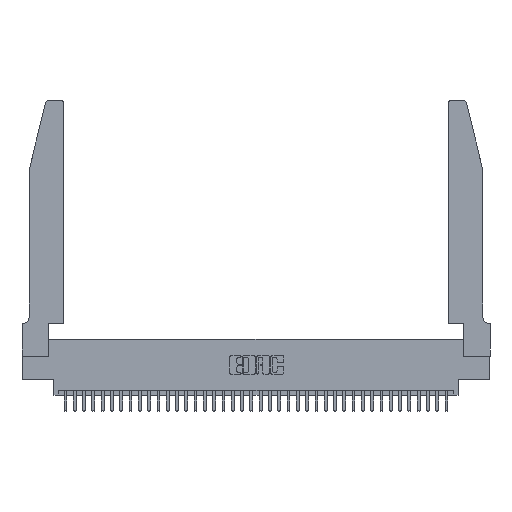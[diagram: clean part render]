
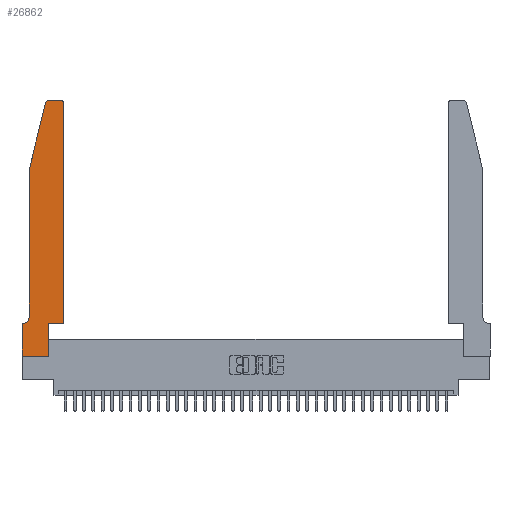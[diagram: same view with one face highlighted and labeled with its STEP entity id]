
A CAD part, top view. The second image highlights one B-rep face of the part: STEP entity #26862.
In plain terms, the highlighted planar face has unit normal (0, 0, 1).
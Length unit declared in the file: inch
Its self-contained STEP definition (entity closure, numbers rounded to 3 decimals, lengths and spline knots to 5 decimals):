
#395 = ORIENTED_EDGE ( 'NONE', *, *, #16836, .T. ) ;
#400 = VERTEX_POINT ( 'NONE', #13882 ) ;
#529 = CARTESIAN_POINT ( 'NONE',  ( 0.0755, 2., 0.37 ) ) ;
#575 = PLANE ( 'NONE',  #10011 ) ;
#700 = DIRECTION ( 'NONE',  ( 1., 0., 0. ) ) ;
#1542 = DIRECTION ( 'NONE',  ( 1., 0., 0. ) ) ;
#2435 = VECTOR ( 'NONE', #3295, 39.37008 ) ;
#2620 = VECTOR ( 'NONE', #33960, 39.37008 ) ;
#2962 = LINE ( 'NONE', #3647, #18760 ) ;
#3295 = DIRECTION ( 'NONE',  ( 0., -1., 0. ) ) ;
#3554 = CARTESIAN_POINT ( 'NONE',  ( 0.0055, 0.42, 0.37 ) ) ;
#3647 = CARTESIAN_POINT ( 'NONE',  ( 0., 0., 0.37 ) ) ;
#4243 = VECTOR ( 'NONE', #6695, 39.37008 ) ;
#4489 = VECTOR ( 'NONE', #28219, 39.37008 ) ;
#5082 = CARTESIAN_POINT ( 'NONE',  ( 0.0755, 0.42, 0.37 ) ) ;
#5367 = LINE ( 'NONE', #30087, #10593 ) ;
#5373 = CARTESIAN_POINT ( 'NONE',  ( 0.4505, 0.35, 0.37 ) ) ;
#5384 = VECTOR ( 'NONE', #25978, 39.37008 ) ;
#5911 = ORIENTED_EDGE ( 'NONE', *, *, #30360, .T. ) ;
#5937 = CARTESIAN_POINT ( 'NONE',  ( 0., 0.35, 0.37 ) ) ;
#6180 = ORIENTED_EDGE ( 'NONE', *, *, #32149, .T. ) ;
#6586 = DIRECTION ( 'NONE',  ( -1., 0., 0. ) ) ;
#6668 = DIRECTION ( 'NONE',  ( 0., -1., 0. ) ) ;
#6695 = DIRECTION ( 'NONE',  ( 0., 1., 0. ) ) ;
#6827 = CARTESIAN_POINT ( 'NONE',  ( 0.4505, 0.35, 0.37 ) ) ;
#6992 = CARTESIAN_POINT ( 'NONE',  ( 0.2865, 0., 0.37 ) ) ;
#8210 = CARTESIAN_POINT ( 'NONE',  ( 0.0755, 2., 0.37 ) ) ;
#8322 = CARTESIAN_POINT ( 'NONE',  ( 0.2865, 0.35, 0.37 ) ) ;
#8502 = VERTEX_POINT ( 'NONE', #5082 ) ;
#8760 = LINE ( 'NONE', #13748, #2620 ) ;
#8770 = CARTESIAN_POINT ( 'NONE',  ( 0., 0., 0.37 ) ) ;
#9893 = AXIS2_PLACEMENT_3D ( 'NONE', #12960, #33146, #15864 ) ;
#9924 = VERTEX_POINT ( 'NONE', #32906 ) ;
#10011 = AXIS2_PLACEMENT_3D ( 'NONE', #29972, #18523, #700 ) ;
#10066 = ORIENTED_EDGE ( 'NONE', *, *, #23446, .T. ) ;
#10461 = VERTEX_POINT ( 'NONE', #5937 ) ;
#10507 = LINE ( 'NONE', #23837, #2435 ) ;
#10521 = VERTEX_POINT ( 'NONE', #29562 ) ;
#10593 = VECTOR ( 'NONE', #27276, 39.37008 ) ;
#10937 = CARTESIAN_POINT ( 'NONE',  ( 0.4505, 0.35, 0.37 ) ) ;
#11650 = ORIENTED_EDGE ( 'NONE', *, *, #18277, .T. ) ;
#11879 = ORIENTED_EDGE ( 'NONE', *, *, #30148, .T. ) ;
#12250 = LINE ( 'NONE', #32814, #4243 ) ;
#12498 = LINE ( 'NONE', #10937, #4489 ) ;
#12588 = VERTEX_POINT ( 'NONE', #6992 ) ;
#12918 = LINE ( 'NONE', #8210, #20580 ) ;
#12960 = CARTESIAN_POINT ( 'NONE',  ( 0.284, 2.72, 0.37 ) ) ;
#13748 = CARTESIAN_POINT ( 'NONE',  ( 0.2605, 2.75, 0.37 ) ) ;
#13882 = CARTESIAN_POINT ( 'NONE',  ( 0., 0., 0.37 ) ) ;
#14014 = CARTESIAN_POINT ( 'NONE',  ( 0.4505, 2.72, 0.37 ) ) ;
#14274 = LINE ( 'NONE', #5373, #5384 ) ;
#14416 = FACE_OUTER_BOUND ( 'NONE', #36557, .T. ) ;
#15118 = VERTEX_POINT ( 'NONE', #31082 ) ;
#15179 = VERTEX_POINT ( 'NONE', #14014 ) ;
#15702 = EDGE_CURVE ( 'NONE', #23972, #27728, #12498, .T. ) ;
#15864 = DIRECTION ( 'NONE',  ( 1., 0., 0. ) ) ;
#16251 = ORIENTED_EDGE ( 'NONE', *, *, #22519, .T. ) ;
#16836 = EDGE_CURVE ( 'NONE', #27728, #15179, #14274, .T. ) ;
#17478 = EDGE_CURVE ( 'NONE', #400, #12588, #36845, .T. ) ;
#18226 = AXIS2_PLACEMENT_3D ( 'NONE', #3554, #24074, #6586 ) ;
#18277 = EDGE_CURVE ( 'NONE', #29444, #8502, #10507, .T. ) ;
#18523 = DIRECTION ( 'NONE',  ( 0., 0., 1. ) ) ;
#18760 = VECTOR ( 'NONE', #6668, 39.37008 ) ;
#19197 = CIRCLE ( 'NONE', #34561, 0.03 ) ;
#19300 = DIRECTION ( 'NONE',  ( 0., 0., 1. ) ) ;
#19609 = ORIENTED_EDGE ( 'NONE', *, *, #23746, .T. ) ;
#20580 = VECTOR ( 'NONE', #25808, 39.37008 ) ;
#22519 = EDGE_CURVE ( 'NONE', #8502, #27505, #29205, .T. ) ;
#23446 = EDGE_CURVE ( 'NONE', #10521, #29444, #12918, .T. ) ;
#23746 = EDGE_CURVE ( 'NONE', #27505, #10461, #5367, .T. ) ;
#23837 = CARTESIAN_POINT ( 'NONE',  ( 0.0755, 2., 0.37 ) ) ;
#23972 = VERTEX_POINT ( 'NONE', #8322 ) ;
#24074 = DIRECTION ( 'NONE',  ( 0., 0., -1. ) ) ;
#24427 = ORIENTED_EDGE ( 'NONE', *, *, #27918, .T. ) ;
#25443 = ORIENTED_EDGE ( 'NONE', *, *, #17478, .T. ) ;
#25808 = DIRECTION ( 'NONE',  ( -0.239, -0.971, 0. ) ) ;
#25978 = DIRECTION ( 'NONE',  ( 0., 1., 0. ) ) ;
#26862 = ADVANCED_FACE ( 'NONE', ( #14416 ), #575, .T. ) ;
#27276 = DIRECTION ( 'NONE',  ( -1., 0., 0. ) ) ;
#27505 = VERTEX_POINT ( 'NONE', #32841 ) ;
#27728 = VERTEX_POINT ( 'NONE', #6827 ) ;
#27918 = EDGE_CURVE ( 'NONE', #15118, #9924, #8760, .T. ) ;
#28201 = ORIENTED_EDGE ( 'NONE', *, *, #32871, .T. ) ;
#28219 = DIRECTION ( 'NONE',  ( 1., 0., 0. ) ) ;
#29205 = CIRCLE ( 'NONE', #18226, 0.07 ) ;
#29444 = VERTEX_POINT ( 'NONE', #529 ) ;
#29562 = CARTESIAN_POINT ( 'NONE',  ( 0.25487, 2.72718, 0.37 ) ) ;
#29972 = CARTESIAN_POINT ( 'NONE',  ( 0., 0.35, 0.37 ) ) ;
#30087 = CARTESIAN_POINT ( 'NONE',  ( 0.0755, 0.35, 0.37 ) ) ;
#30148 = EDGE_CURVE ( 'NONE', #10461, #400, #2962, .T. ) ;
#30360 = EDGE_CURVE ( 'NONE', #15179, #15118, #19197, .T. ) ;
#30411 = ORIENTED_EDGE ( 'NONE', *, *, #15702, .T. ) ;
#31082 = CARTESIAN_POINT ( 'NONE',  ( 0.4205, 2.75, 0.37 ) ) ;
#32149 = EDGE_CURVE ( 'NONE', #12588, #23972, #12250, .T. ) ;
#32814 = CARTESIAN_POINT ( 'NONE',  ( 0.2865, 0.35, 0.37 ) ) ;
#32841 = CARTESIAN_POINT ( 'NONE',  ( 0.0055, 0.35, 0.37 ) ) ;
#32871 = EDGE_CURVE ( 'NONE', #9924, #10521, #33888, .T. ) ;
#32906 = CARTESIAN_POINT ( 'NONE',  ( 0.284, 2.75, 0.37 ) ) ;
#33146 = DIRECTION ( 'NONE',  ( 0., 0., 1. ) ) ;
#33888 = CIRCLE ( 'NONE', #9893, 0.03 ) ;
#33960 = DIRECTION ( 'NONE',  ( -1., 0., 0. ) ) ;
#34561 = AXIS2_PLACEMENT_3D ( 'NONE', #36608, #19300, #1542 ) ;
#34929 = DIRECTION ( 'NONE',  ( 1., 0., 0. ) ) ;
#35918 = VECTOR ( 'NONE', #34929, 39.37008 ) ;
#36557 = EDGE_LOOP ( 'NONE', ( #24427, #28201, #10066, #11650, #16251, #19609, #11879, #25443, #6180, #30411, #395, #5911 ) ) ;
#36608 = CARTESIAN_POINT ( 'NONE',  ( 0.4205, 2.72, 0.37 ) ) ;
#36845 = LINE ( 'NONE', #8770, #35918 ) ;
